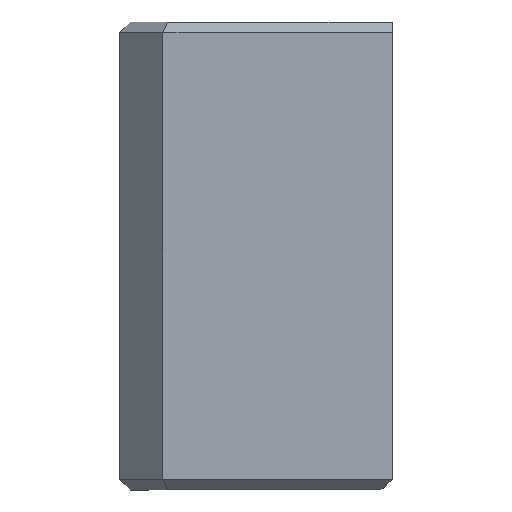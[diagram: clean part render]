
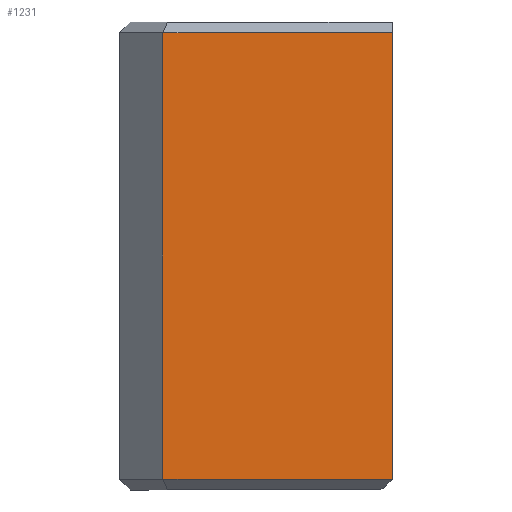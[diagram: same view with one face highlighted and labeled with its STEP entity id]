
A CAD part, left-side view. The second image highlights one B-rep face of the part: STEP entity #1231.
In plain terms, the highlighted planar face has unit normal (-1, 0, 0).
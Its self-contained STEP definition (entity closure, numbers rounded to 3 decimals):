
#121=FACE_OUTER_BOUND('',#194,.T.);
#194=EDGE_LOOP('',(#873,#874,#875,#876));
#265=LINE('',#1589,#389);
#291=LINE('',#1749,#415);
#294=LINE('',#1755,#418);
#295=LINE('',#1756,#419);
#389=VECTOR('',#1363,10.);
#415=VECTOR('',#1401,10.);
#418=VECTOR('',#1406,10.);
#419=VECTOR('',#1407,10.);
#513=VERTEX_POINT('',#1587);
#514=VERTEX_POINT('',#1588);
#552=VERTEX_POINT('',#1748);
#554=VERTEX_POINT('',#1754);
#631=EDGE_CURVE('',#513,#514,#265,.T.);
#675=EDGE_CURVE('',#552,#514,#291,.T.);
#678=EDGE_CURVE('',#513,#554,#294,.T.);
#679=EDGE_CURVE('',#552,#554,#295,.T.);
#873=ORIENTED_EDGE('',*,*,#631,.F.);
#874=ORIENTED_EDGE('',*,*,#678,.T.);
#875=ORIENTED_EDGE('',*,*,#679,.F.);
#876=ORIENTED_EDGE('',*,*,#675,.T.);
#1190=PLANE('',#1316);
#1231=ADVANCED_FACE('',(#121),#1190,.T.);
#1316=AXIS2_PLACEMENT_3D('',#1753,#1404,#1405);
#1363=DIRECTION('',(0.,-1.,0.));
#1401=DIRECTION('',(0.,0.,1.));
#1404=DIRECTION('center_axis',(-1.,0.,0.));
#1405=DIRECTION('ref_axis',(0.,-1.,0.));
#1406=DIRECTION('',(0.,0.,-1.));
#1407=DIRECTION('',(0.,1.,0.));
#1587=CARTESIAN_POINT('',(105.851,21.852,43.5));
#1588=CARTESIAN_POINT('',(105.851,0.051,43.5));
#1589=CARTESIAN_POINT('',(105.851,18.061,43.5));
#1748=CARTESIAN_POINT('',(105.851,0.051,1.));
#1749=CARTESIAN_POINT('',(105.851,0.051,0.));
#1753=CARTESIAN_POINT('Origin',(105.851,23.114,0.));
#1754=CARTESIAN_POINT('',(105.851,21.852,1.));
#1755=CARTESIAN_POINT('',(105.851,21.852,0.));
#1756=CARTESIAN_POINT('',(105.851,18.061,1.));
